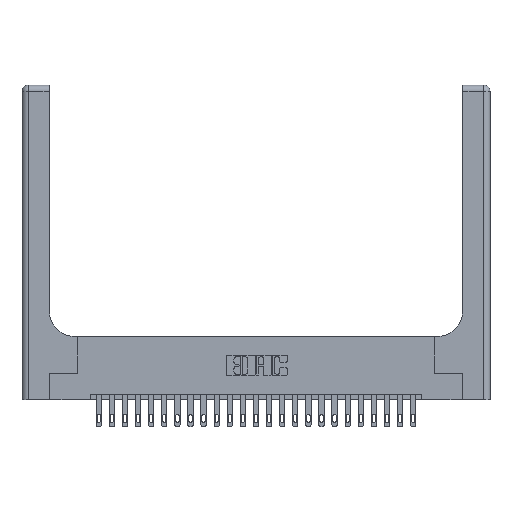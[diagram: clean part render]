
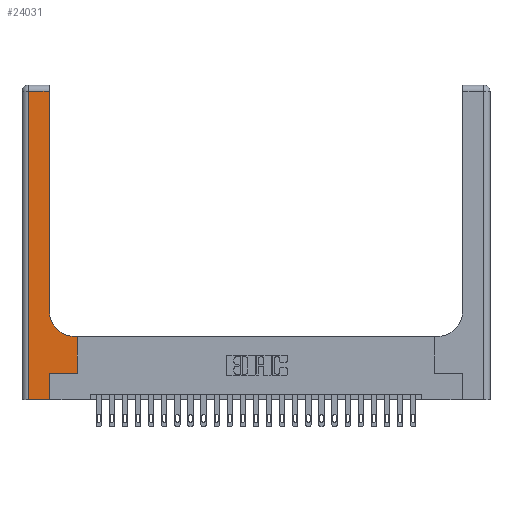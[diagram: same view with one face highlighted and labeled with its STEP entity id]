
A CAD part, top view. The second image highlights one B-rep face of the part: STEP entity #24031.
In plain terms, the highlighted planar face has unit normal (0, 0, 1).
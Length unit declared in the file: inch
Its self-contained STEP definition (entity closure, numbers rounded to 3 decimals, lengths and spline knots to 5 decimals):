
#492 = VERTEX_POINT ( 'NONE', #1252 ) ;
#977 = VERTEX_POINT ( 'NONE', #19828 ) ;
#1126 = ORIENTED_EDGE ( 'NONE', *, *, #3303, .T. ) ;
#1252 = CARTESIAN_POINT ( 'NONE',  ( 0.265, 0., 0.37 ) ) ;
#1408 = CARTESIAN_POINT ( 'NONE',  ( 0., 2.94, 0.37 ) ) ;
#1851 = VECTOR ( 'NONE', #4708, 39.37008 ) ;
#1871 = VECTOR ( 'NONE', #21512, 39.37008 ) ;
#1990 = LINE ( 'NONE', #7621, #5132 ) ;
#2430 = AXIS2_PLACEMENT_3D ( 'NONE', #9631, #16855, #9871 ) ;
#2522 = VECTOR ( 'NONE', #16813, 39.37008 ) ;
#2544 = EDGE_CURVE ( 'NONE', #977, #15846, #20917, .T. ) ;
#2947 = CARTESIAN_POINT ( 'NONE',  ( 0.51, 0.6, 0.37 ) ) ;
#3085 = VERTEX_POINT ( 'NONE', #19415 ) ;
#3303 = EDGE_CURVE ( 'NONE', #15834, #10988, #18147, .T. ) ;
#3552 = VECTOR ( 'NONE', #18252, 39.37008 ) ;
#3647 = PLANE ( 'NONE',  #11639 ) ;
#4140 = VERTEX_POINT ( 'NONE', #2947 ) ;
#4593 = CARTESIAN_POINT ( 'NONE',  ( 0.528, 0.25, 0.37 ) ) ;
#4708 = DIRECTION ( 'NONE',  ( -1., 0., 0. ) ) ;
#5132 = VECTOR ( 'NONE', #15093, 39.37008 ) ;
#5389 = ORIENTED_EDGE ( 'NONE', *, *, #5399, .T. ) ;
#5399 = EDGE_CURVE ( 'NONE', #492, #977, #10766, .T. ) ;
#6342 = CIRCLE ( 'NONE', #2430, 0.25 ) ;
#6362 = EDGE_CURVE ( 'NONE', #10988, #492, #1990, .T. ) ;
#7263 = EDGE_CURVE ( 'NONE', #4140, #22935, #6342, .T. ) ;
#7621 = CARTESIAN_POINT ( 'NONE',  ( 0., 0., 0.37 ) ) ;
#7994 = LINE ( 'NONE', #17419, #15369 ) ;
#8919 = DIRECTION ( 'NONE',  ( 0., 0., -1. ) ) ;
#8936 = CARTESIAN_POINT ( 'NONE',  ( 0.06, 0., 0.37 ) ) ;
#9342 = CARTESIAN_POINT ( 'NONE',  ( 0.26, 3., 0.37 ) ) ;
#9631 = CARTESIAN_POINT ( 'NONE',  ( 0.51, 0.85, 0.37 ) ) ;
#9806 = CARTESIAN_POINT ( 'NONE',  ( 0.528, 0.25, 0.37 ) ) ;
#9871 = DIRECTION ( 'NONE',  ( 1., 0., 0. ) ) ;
#10745 = FACE_OUTER_BOUND ( 'NONE', #18494, .T. ) ;
#10766 = LINE ( 'NONE', #20569, #3552 ) ;
#10988 = VERTEX_POINT ( 'NONE', #8936 ) ;
#11521 = DIRECTION ( 'NONE',  ( 0., -1., 0. ) ) ;
#11540 = DIRECTION ( 'NONE',  ( -1., 0., 0. ) ) ;
#11639 = AXIS2_PLACEMENT_3D ( 'NONE', #22133, #8919, #16389 ) ;
#11922 = ORIENTED_EDGE ( 'NONE', *, *, #2544, .T. ) ;
#12227 = VERTEX_POINT ( 'NONE', #17368 ) ;
#12493 = ORIENTED_EDGE ( 'NONE', *, *, #16091, .T. ) ;
#12922 = CARTESIAN_POINT ( 'NONE',  ( 0.26, 0.85, 0.37 ) ) ;
#13253 = LINE ( 'NONE', #9806, #21602 ) ;
#15093 = DIRECTION ( 'NONE',  ( 1., 0., 0. ) ) ;
#15369 = VECTOR ( 'NONE', #11540, 39.37008 ) ;
#15549 = ORIENTED_EDGE ( 'NONE', *, *, #18743, .T. ) ;
#15834 = VERTEX_POINT ( 'NONE', #17811 ) ;
#15846 = VERTEX_POINT ( 'NONE', #4593 ) ;
#16091 = EDGE_CURVE ( 'NONE', #15846, #12227, #13253, .T. ) ;
#16389 = DIRECTION ( 'NONE',  ( -1., 0., 0. ) ) ;
#16813 = DIRECTION ( 'NONE',  ( 0., 1., 0. ) ) ;
#16855 = DIRECTION ( 'NONE',  ( 0., 0., -1. ) ) ;
#17368 = CARTESIAN_POINT ( 'NONE',  ( 0.528, 0.6, 0.37 ) ) ;
#17419 = CARTESIAN_POINT ( 'NONE',  ( 0.26, 0.6, 0.37 ) ) ;
#17811 = CARTESIAN_POINT ( 'NONE',  ( 0.06, 2.94, 0.37 ) ) ;
#18147 = LINE ( 'NONE', #23768, #23237 ) ;
#18252 = DIRECTION ( 'NONE',  ( 0., 1., 0. ) ) ;
#18467 = CARTESIAN_POINT ( 'NONE',  ( 0.265, 0.25, 0.37 ) ) ;
#18494 = EDGE_LOOP ( 'NONE', ( #22751, #21933, #1126, #21169, #5389, #11922, #12493, #15549, #23476 ) ) ;
#18743 = EDGE_CURVE ( 'NONE', #12227, #4140, #7994, .T. ) ;
#19415 = CARTESIAN_POINT ( 'NONE',  ( 0.26, 2.94, 0.37 ) ) ;
#19828 = CARTESIAN_POINT ( 'NONE',  ( 0.265, 0.25, 0.37 ) ) ;
#20332 = EDGE_CURVE ( 'NONE', #22935, #3085, #20511, .T. ) ;
#20511 = LINE ( 'NONE', #9342, #2522 ) ;
#20569 = CARTESIAN_POINT ( 'NONE',  ( 0.265, 0., 0.37 ) ) ;
#20726 = DIRECTION ( 'NONE',  ( 0., 1., 0. ) ) ;
#20917 = LINE ( 'NONE', #18467, #1871 ) ;
#21169 = ORIENTED_EDGE ( 'NONE', *, *, #6362, .T. ) ;
#21482 = LINE ( 'NONE', #1408, #1851 ) ;
#21512 = DIRECTION ( 'NONE',  ( 1., 0., 0. ) ) ;
#21602 = VECTOR ( 'NONE', #20726, 39.37008 ) ;
#21933 = ORIENTED_EDGE ( 'NONE', *, *, #23166, .T. ) ;
#22133 = CARTESIAN_POINT ( 'NONE',  ( 0., 3., 0.37 ) ) ;
#22751 = ORIENTED_EDGE ( 'NONE', *, *, #20332, .T. ) ;
#22935 = VERTEX_POINT ( 'NONE', #12922 ) ;
#23166 = EDGE_CURVE ( 'NONE', #3085, #15834, #21482, .T. ) ;
#23237 = VECTOR ( 'NONE', #11521, 39.37008 ) ;
#23476 = ORIENTED_EDGE ( 'NONE', *, *, #7263, .T. ) ;
#23768 = CARTESIAN_POINT ( 'NONE',  ( 0.06, 3., 0.37 ) ) ;
#24031 = ADVANCED_FACE ( 'NONE', ( #10745 ), #3647, .F. ) ;
